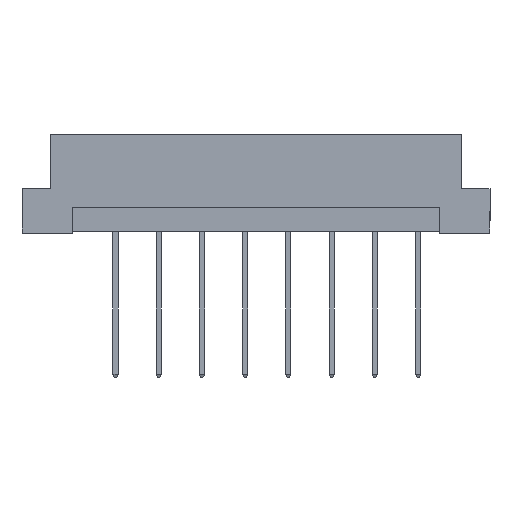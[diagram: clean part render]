
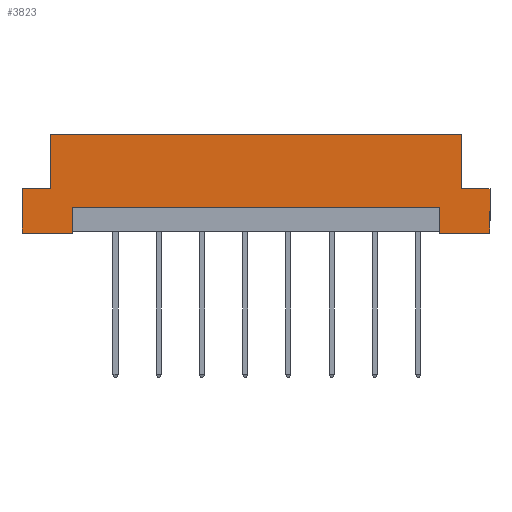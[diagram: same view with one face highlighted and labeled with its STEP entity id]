
A CAD part, front view. The second image highlights one B-rep face of the part: STEP entity #3823.
In plain terms, the highlighted planar face has unit normal (0, -1, 0).
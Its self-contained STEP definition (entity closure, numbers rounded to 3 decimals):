
#96 = VECTOR ( 'NONE', #4883, 1000. ) ;
#134 = LINE ( 'NONE', #570, #3246 ) ;
#199 = CARTESIAN_POINT ( 'NONE',  ( -21.6, -4.3, 0.2 ) ) ;
#278 = DIRECTION ( 'NONE',  ( 1., 0., 0. ) ) ;
#282 = VERTEX_POINT ( 'NONE', #4059 ) ;
#477 = CARTESIAN_POINT ( 'NONE',  ( -27.5, -4.3, 5.2 ) ) ;
#512 = VECTOR ( 'NONE', #1411, 1000. ) ;
#540 = VECTOR ( 'NONE', #278, 1000. ) ;
#550 = CARTESIAN_POINT ( 'NONE',  ( -27.5, -4.3, 11.6 ) ) ;
#570 = CARTESIAN_POINT ( 'NONE',  ( -21.6, -4.3, 3. ) ) ;
#668 = CARTESIAN_POINT ( 'NONE',  ( 27.5, -4.3, 0. ) ) ;
#749 = VECTOR ( 'NONE', #860, 1000. ) ;
#860 = DIRECTION ( 'NONE',  ( 1., 0., 0. ) ) ;
#980 = LINE ( 'NONE', #2033, #6346 ) ;
#1024 = EDGE_LOOP ( 'NONE', ( #3901, #6170, #1770, #4594, #6107, #5567, #5835, #4474, #5419, #6372, #3826, #5225 ) ) ;
#1066 = VERTEX_POINT ( 'NONE', #477 ) ;
#1148 = EDGE_CURVE ( 'NONE', #282, #5490, #6664, .T. ) ;
#1153 = LINE ( 'NONE', #199, #96 ) ;
#1155 = VECTOR ( 'NONE', #3529, 1000. ) ;
#1180 = DIRECTION ( 'NONE',  ( 0., 1., 0. ) ) ;
#1193 = EDGE_CURVE ( 'NONE', #4723, #2069, #5660, .T. ) ;
#1212 = CARTESIAN_POINT ( 'NONE',  ( 27.5, -4.3, 11.6 ) ) ;
#1233 = EDGE_CURVE ( 'NONE', #1066, #6171, #4717, .T. ) ;
#1317 = CARTESIAN_POINT ( 'NONE',  ( -21.6, -4.3, 3. ) ) ;
#1391 = EDGE_CURVE ( 'NONE', #6171, #1647, #2825, .T. ) ;
#1411 = DIRECTION ( 'NONE',  ( 1., 0., 0. ) ) ;
#1449 = CARTESIAN_POINT ( 'NONE',  ( 24.2, -4.3, 11.6 ) ) ;
#1647 = VERTEX_POINT ( 'NONE', #2527 ) ;
#1770 = ORIENTED_EDGE ( 'NONE', *, *, #4127, .T. ) ;
#1907 = VERTEX_POINT ( 'NONE', #1317 ) ;
#2033 = CARTESIAN_POINT ( 'NONE',  ( -24.2, -4.3, 5.2 ) ) ;
#2069 = VERTEX_POINT ( 'NONE', #1449 ) ;
#2096 = EDGE_CURVE ( 'NONE', #2988, #3560, #980, .T. ) ;
#2153 = AXIS2_PLACEMENT_3D ( 'NONE', #1212, #1180, #3193 ) ;
#2355 = VERTEX_POINT ( 'NONE', #668 ) ;
#2527 = CARTESIAN_POINT ( 'NONE',  ( -21.6, -4.3, 0. ) ) ;
#2825 = LINE ( 'NONE', #5421, #3116 ) ;
#2882 = DIRECTION ( 'NONE',  ( 1., 0., 0. ) ) ;
#2893 = CARTESIAN_POINT ( 'NONE',  ( 27.5, -4.3, 11.6 ) ) ;
#2928 = LINE ( 'NONE', #6063, #4527 ) ;
#2960 = DIRECTION ( 'NONE',  ( 0., 0., -1. ) ) ;
#2988 = VERTEX_POINT ( 'NONE', #4907 ) ;
#3005 = CARTESIAN_POINT ( 'NONE',  ( 27.5, -4.3, 0. ) ) ;
#3026 = VECTOR ( 'NONE', #5932, 1000. ) ;
#3100 = CARTESIAN_POINT ( 'NONE',  ( 24.2, -4.3, 5.2 ) ) ;
#3116 = VECTOR ( 'NONE', #2882, 1000. ) ;
#3193 = DIRECTION ( 'NONE',  ( -1., 0., 0. ) ) ;
#3246 = VECTOR ( 'NONE', #5312, 1000. ) ;
#3391 = CARTESIAN_POINT ( 'NONE',  ( -27.5, -4.3, 0. ) ) ;
#3395 = CARTESIAN_POINT ( 'NONE',  ( -27.5, -4.3, 5.2 ) ) ;
#3529 = DIRECTION ( 'NONE',  ( 0., 0., 1. ) ) ;
#3560 = VERTEX_POINT ( 'NONE', #4399 ) ;
#3647 = FACE_OUTER_BOUND ( 'NONE', #1024, .T. ) ;
#3746 = VECTOR ( 'NONE', #5155, 1000. ) ;
#3823 = ADVANCED_FACE ( 'NONE', ( #3647 ), #6289, .F. ) ;
#3826 = ORIENTED_EDGE ( 'NONE', *, *, #1391, .T. ) ;
#3901 = ORIENTED_EDGE ( 'NONE', *, *, #5159, .T. ) ;
#4051 = LINE ( 'NONE', #3005, #512 ) ;
#4059 = CARTESIAN_POINT ( 'NONE',  ( 21.6, -4.3, 0. ) ) ;
#4088 = DIRECTION ( 'NONE',  ( 0., 0., 1. ) ) ;
#4127 = EDGE_CURVE ( 'NONE', #282, #2355, #4051, .T. ) ;
#4141 = CARTESIAN_POINT ( 'NONE',  ( 21.6, -4.3, 0.2 ) ) ;
#4256 = CARTESIAN_POINT ( 'NONE',  ( 21.6, -4.3, 3. ) ) ;
#4399 = CARTESIAN_POINT ( 'NONE',  ( -24.2, -4.3, 11.6 ) ) ;
#4402 = EDGE_CURVE ( 'NONE', #4723, #6688, #4923, .T. ) ;
#4474 = ORIENTED_EDGE ( 'NONE', *, *, #2096, .F. ) ;
#4527 = VECTOR ( 'NONE', #2960, 1000. ) ;
#4594 = ORIENTED_EDGE ( 'NONE', *, *, #6266, .F. ) ;
#4671 = EDGE_CURVE ( 'NONE', #1907, #1647, #1153, .T. ) ;
#4717 = LINE ( 'NONE', #550, #5371 ) ;
#4723 = VERTEX_POINT ( 'NONE', #6383 ) ;
#4883 = DIRECTION ( 'NONE',  ( 0., 0., -1. ) ) ;
#4885 = CARTESIAN_POINT ( 'NONE',  ( 27.5, -4.3, 5.2 ) ) ;
#4907 = CARTESIAN_POINT ( 'NONE',  ( -24.2, -4.3, 5.2 ) ) ;
#4923 = LINE ( 'NONE', #5866, #3026 ) ;
#4961 = LINE ( 'NONE', #3395, #749 ) ;
#5155 = DIRECTION ( 'NONE',  ( 0., 0., 1. ) ) ;
#5159 = EDGE_CURVE ( 'NONE', #1907, #5490, #134, .T. ) ;
#5225 = ORIENTED_EDGE ( 'NONE', *, *, #4671, .F. ) ;
#5312 = DIRECTION ( 'NONE',  ( 1., 0., 0. ) ) ;
#5371 = VECTOR ( 'NONE', #6327, 1000. ) ;
#5419 = ORIENTED_EDGE ( 'NONE', *, *, #5638, .F. ) ;
#5421 = CARTESIAN_POINT ( 'NONE',  ( 27.5, -4.3, 0. ) ) ;
#5490 = VERTEX_POINT ( 'NONE', #4256 ) ;
#5567 = ORIENTED_EDGE ( 'NONE', *, *, #1193, .T. ) ;
#5638 = EDGE_CURVE ( 'NONE', #1066, #2988, #4961, .T. ) ;
#5657 = EDGE_CURVE ( 'NONE', #3560, #2069, #5891, .T. ) ;
#5660 = LINE ( 'NONE', #3100, #3746 ) ;
#5835 = ORIENTED_EDGE ( 'NONE', *, *, #5657, .F. ) ;
#5866 = CARTESIAN_POINT ( 'NONE',  ( 27.5, -4.3, 5.2 ) ) ;
#5891 = LINE ( 'NONE', #2893, #540 ) ;
#5932 = DIRECTION ( 'NONE',  ( 1., 0., 0. ) ) ;
#6063 = CARTESIAN_POINT ( 'NONE',  ( 27.5, -4.3, 11.6 ) ) ;
#6107 = ORIENTED_EDGE ( 'NONE', *, *, #4402, .F. ) ;
#6170 = ORIENTED_EDGE ( 'NONE', *, *, #1148, .F. ) ;
#6171 = VERTEX_POINT ( 'NONE', #3391 ) ;
#6266 = EDGE_CURVE ( 'NONE', #6688, #2355, #2928, .T. ) ;
#6289 = PLANE ( 'NONE',  #2153 ) ;
#6327 = DIRECTION ( 'NONE',  ( 0., 0., -1. ) ) ;
#6346 = VECTOR ( 'NONE', #4088, 1000. ) ;
#6372 = ORIENTED_EDGE ( 'NONE', *, *, #1233, .T. ) ;
#6383 = CARTESIAN_POINT ( 'NONE',  ( 24.2, -4.3, 5.2 ) ) ;
#6664 = LINE ( 'NONE', #4141, #1155 ) ;
#6688 = VERTEX_POINT ( 'NONE', #4885 ) ;
